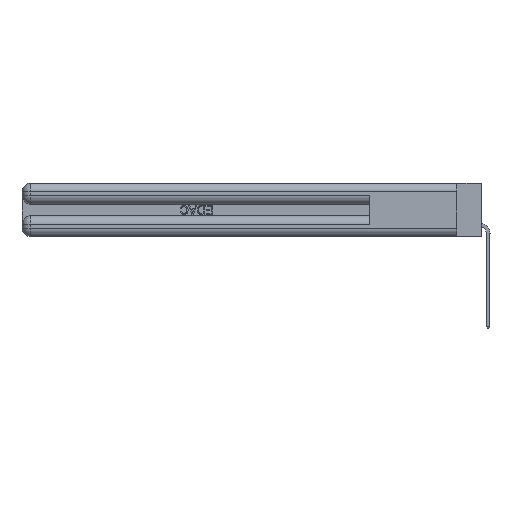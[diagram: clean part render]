
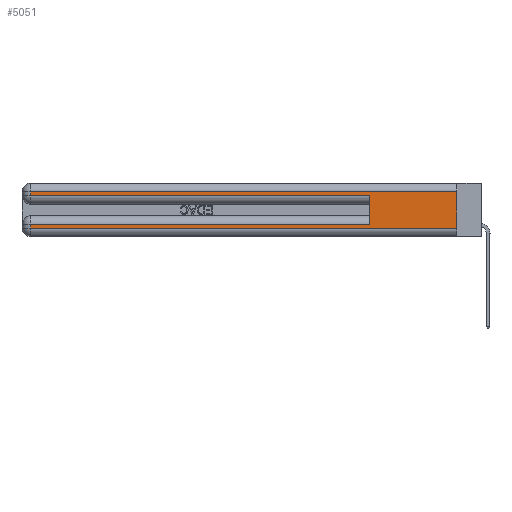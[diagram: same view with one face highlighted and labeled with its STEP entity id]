
A CAD part, left-side view. The second image highlights one B-rep face of the part: STEP entity #5051.
In plain terms, the highlighted planar face has unit normal (-1, 0, 0).
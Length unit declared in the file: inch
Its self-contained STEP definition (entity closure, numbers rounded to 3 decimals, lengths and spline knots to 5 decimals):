
#98 = CARTESIAN_POINT ( 'NONE',  ( 0., 0., 0.37 ) ) ;
#243 = LINE ( 'NONE', #23332, #40090 ) ;
#339 = ORIENTED_EDGE ( 'NONE', *, *, #33519, .T. ) ;
#570 = EDGE_CURVE ( 'NONE', #37693, #42604, #21354, .T. ) ;
#928 = EDGE_CURVE ( 'NONE', #13161, #44256, #34047, .T. ) ;
#1303 = EDGE_CURVE ( 'NONE', #37693, #14995, #27836, .T. ) ;
#2771 = DIRECTION ( 'NONE',  ( 0., 1., 0. ) ) ;
#3170 = DIRECTION ( 'NONE',  ( 0., 0., 1. ) ) ;
#3204 = CARTESIAN_POINT ( 'NONE',  ( 0., 0.6, 0.085 ) ) ;
#4733 = DIRECTION ( 'NONE',  ( 1., 0., 0. ) ) ;
#5051 = ADVANCED_FACE ( 'NONE', ( #9451 ), #23177, .F. ) ;
#5146 = VERTEX_POINT ( 'NONE', #26723 ) ;
#6179 = EDGE_CURVE ( 'NONE', #44256, #16551, #34167, .T. ) ;
#8031 = CARTESIAN_POINT ( 'NONE',  ( 0., 0., 0.37 ) ) ;
#9035 = EDGE_CURVE ( 'NONE', #13161, #5146, #16692, .T. ) ;
#9308 = CARTESIAN_POINT ( 'NONE',  ( 0., 0., 0.085 ) ) ;
#9451 = FACE_OUTER_BOUND ( 'NONE', #43398, .T. ) ;
#10751 = LINE ( 'NONE', #49691, #48121 ) ;
#13161 = VERTEX_POINT ( 'NONE', #3204 ) ;
#13226 = VERTEX_POINT ( 'NONE', #23157 ) ;
#14995 = VERTEX_POINT ( 'NONE', #22041 ) ;
#15009 = VECTOR ( 'NONE', #3170, 39.37008 ) ;
#15534 = ORIENTED_EDGE ( 'NONE', *, *, #43748, .T. ) ;
#16110 = DIRECTION ( 'NONE',  ( 0., 0., -1. ) ) ;
#16146 = CARTESIAN_POINT ( 'NONE',  ( 0., 0., 0.31 ) ) ;
#16551 = VERTEX_POINT ( 'NONE', #34504 ) ;
#16692 = LINE ( 'NONE', #29622, #15009 ) ;
#18852 = VECTOR ( 'NONE', #48330, 39.37008 ) ;
#18941 = VECTOR ( 'NONE', #16110, 39.37008 ) ;
#20847 = EDGE_CURVE ( 'NONE', #14995, #13226, #28384, .T. ) ;
#21354 = LINE ( 'NONE', #8031, #18941 ) ;
#22041 = CARTESIAN_POINT ( 'NONE',  ( 0., 2.94, 0.31 ) ) ;
#23157 = CARTESIAN_POINT ( 'NONE',  ( 0., 2.94, 0.285 ) ) ;
#23177 = PLANE ( 'NONE',  #47712 ) ;
#23332 = CARTESIAN_POINT ( 'NONE',  ( 0., 0., 0.06 ) ) ;
#26723 = CARTESIAN_POINT ( 'NONE',  ( 0., 0.6, 0.285 ) ) ;
#27530 = DIRECTION ( 'NONE',  ( 0., -1., 0. ) ) ;
#27836 = LINE ( 'NONE', #48137, #18852 ) ;
#28146 = CARTESIAN_POINT ( 'NONE',  ( 0., 2.94, 0.37 ) ) ;
#28384 = LINE ( 'NONE', #29996, #38114 ) ;
#29607 = DIRECTION ( 'NONE',  ( 0., -1., 0. ) ) ;
#29622 = CARTESIAN_POINT ( 'NONE',  ( 0., 0.6, 0.145 ) ) ;
#29800 = VECTOR ( 'NONE', #2771, 39.37008 ) ;
#29996 = CARTESIAN_POINT ( 'NONE',  ( 0., 2.94, 0.37 ) ) ;
#30956 = ORIENTED_EDGE ( 'NONE', *, *, #9035, .F. ) ;
#32810 = ORIENTED_EDGE ( 'NONE', *, *, #570, .F. ) ;
#32918 = VECTOR ( 'NONE', #39978, 39.37008 ) ;
#33519 = EDGE_CURVE ( 'NONE', #16551, #42604, #243, .T. ) ;
#34047 = LINE ( 'NONE', #9308, #29800 ) ;
#34167 = LINE ( 'NONE', #28146, #32918 ) ;
#34504 = CARTESIAN_POINT ( 'NONE',  ( 0., 2.94, 0.06 ) ) ;
#34737 = DIRECTION ( 'NONE',  ( 0., 0., -1. ) ) ;
#37177 = ORIENTED_EDGE ( 'NONE', *, *, #1303, .T. ) ;
#37513 = CARTESIAN_POINT ( 'NONE',  ( 0., 2.94, 0.085 ) ) ;
#37693 = VERTEX_POINT ( 'NONE', #16146 ) ;
#38072 = ORIENTED_EDGE ( 'NONE', *, *, #20847, .T. ) ;
#38114 = VECTOR ( 'NONE', #34737, 39.37008 ) ;
#38162 = CARTESIAN_POINT ( 'NONE',  ( 0., 0., 0.06 ) ) ;
#39978 = DIRECTION ( 'NONE',  ( 0., 0., -1. ) ) ;
#40090 = VECTOR ( 'NONE', #27530, 39.37008 ) ;
#42604 = VERTEX_POINT ( 'NONE', #38162 ) ;
#43398 = EDGE_LOOP ( 'NONE', ( #32810, #37177, #38072, #15534, #30956, #47265, #44686, #339 ) ) ;
#43748 = EDGE_CURVE ( 'NONE', #13226, #5146, #10751, .T. ) ;
#44256 = VERTEX_POINT ( 'NONE', #37513 ) ;
#44686 = ORIENTED_EDGE ( 'NONE', *, *, #6179, .T. ) ;
#47265 = ORIENTED_EDGE ( 'NONE', *, *, #928, .T. ) ;
#47712 = AXIS2_PLACEMENT_3D ( 'NONE', #98, #4733, #48691 ) ;
#48121 = VECTOR ( 'NONE', #29607, 39.37008 ) ;
#48137 = CARTESIAN_POINT ( 'NONE',  ( 0., 0., 0.31 ) ) ;
#48330 = DIRECTION ( 'NONE',  ( 0., 1., 0. ) ) ;
#48691 = DIRECTION ( 'NONE',  ( 0., 0., -1. ) ) ;
#49691 = CARTESIAN_POINT ( 'NONE',  ( 0., 0., 0.285 ) ) ;
